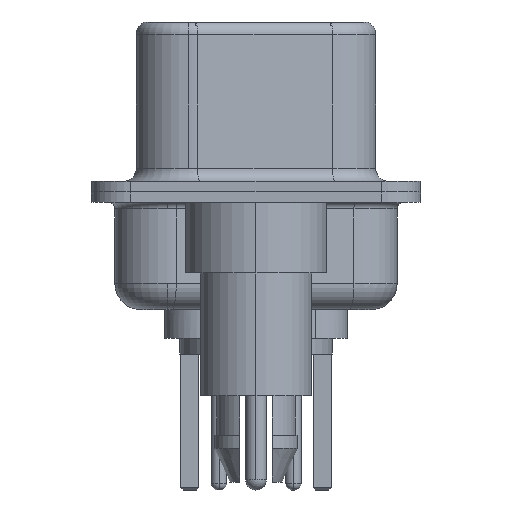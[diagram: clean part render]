
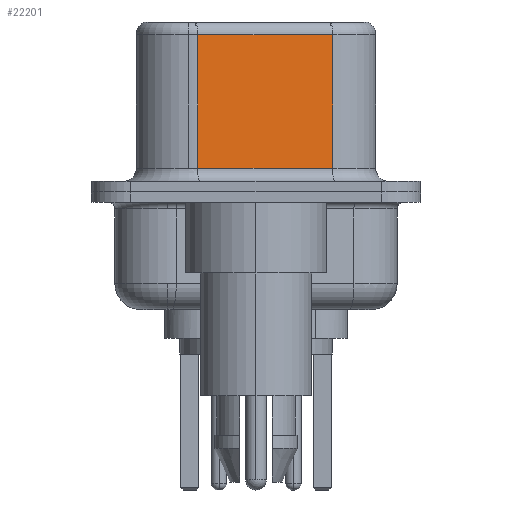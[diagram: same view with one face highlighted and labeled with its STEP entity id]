
A CAD part, left-side view. The second image highlights one B-rep face of the part: STEP entity #22201.
In plain terms, the highlighted planar face has unit normal (-0.985, -0.174, 0).
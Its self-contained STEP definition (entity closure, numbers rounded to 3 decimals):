
#36 = LINE ( 'NONE', #22256, #23264 ) ;
#1832 = DIRECTION ( 'NONE',  ( 0.174, -0.985, 0. ) ) ;
#2345 = DIRECTION ( 'NONE',  ( -0.174, 0.985, 0. ) ) ;
#2414 = CARTESIAN_POINT ( 'NONE',  ( 4.58, -2.927, 6.02 ) ) ;
#2954 = VECTOR ( 'NONE', #25059, 1000. ) ;
#2990 = EDGE_CURVE ( 'NONE', #13651, #9610, #15715, .T. ) ;
#5120 = DIRECTION ( 'NONE',  ( 0.985, 0.174, 0. ) ) ;
#5304 = ORIENTED_EDGE ( 'NONE', *, *, #24586, .T. ) ;
#9029 = CARTESIAN_POINT ( 'NONE',  ( 3.67, 2.233, 6.02 ) ) ;
#9610 = VERTEX_POINT ( 'NONE', #13912 ) ;
#10988 = EDGE_CURVE ( 'NONE', #19596, #26270, #36, .T. ) ;
#11905 = CARTESIAN_POINT ( 'NONE',  ( 4.58, -2.927, 6.02 ) ) ;
#12987 = EDGE_CURVE ( 'NONE', #13651, #19596, #19414, .T. ) ;
#13020 = VECTOR ( 'NONE', #2345, 1000. ) ;
#13651 = VERTEX_POINT ( 'NONE', #2414 ) ;
#13683 = ORIENTED_EDGE ( 'NONE', *, *, #10988, .T. ) ;
#13912 = CARTESIAN_POINT ( 'NONE',  ( 4.58, -2.927, 0.9 ) ) ;
#15145 = CARTESIAN_POINT ( 'NONE',  ( 3.67, 2.233, 0.9 ) ) ;
#15715 = LINE ( 'NONE', #17881, #2954 ) ;
#17881 = CARTESIAN_POINT ( 'NONE',  ( 4.58, -2.927, 6.52 ) ) ;
#18592 = CARTESIAN_POINT ( 'NONE',  ( 4.58, -2.927, 0.9 ) ) ;
#19190 = VECTOR ( 'NONE', #1832, 1000. ) ;
#19414 = LINE ( 'NONE', #11905, #13020 ) ;
#19460 = PLANE ( 'NONE',  #24201 ) ;
#19596 = VERTEX_POINT ( 'NONE', #9029 ) ;
#19945 = LINE ( 'NONE', #18592, #19190 ) ;
#20336 = ORIENTED_EDGE ( 'NONE', *, *, #2990, .F. ) ;
#21564 = FACE_OUTER_BOUND ( 'NONE', #22171, .T. ) ;
#21847 = DIRECTION ( 'NONE',  ( -0.174, 0.985, 0. ) ) ;
#22171 = EDGE_LOOP ( 'NONE', ( #20336, #25808, #13683, #5304 ) ) ;
#22201 = ADVANCED_FACE ( 'NONE', ( #21564 ), #19460, .F. ) ;
#22256 = CARTESIAN_POINT ( 'NONE',  ( 3.67, 2.233, 6.52 ) ) ;
#23264 = VECTOR ( 'NONE', #24614, 1000. ) ;
#24201 = AXIS2_PLACEMENT_3D ( 'NONE', #26479, #5120, #21847 ) ;
#24586 = EDGE_CURVE ( 'NONE', #26270, #9610, #19945, .T. ) ;
#24614 = DIRECTION ( 'NONE',  ( 0., 0., -1. ) ) ;
#25059 = DIRECTION ( 'NONE',  ( 0., 0., -1. ) ) ;
#25808 = ORIENTED_EDGE ( 'NONE', *, *, #12987, .T. ) ;
#26270 = VERTEX_POINT ( 'NONE', #15145 ) ;
#26479 = CARTESIAN_POINT ( 'NONE',  ( 4.58, -2.927, 6.52 ) ) ;
